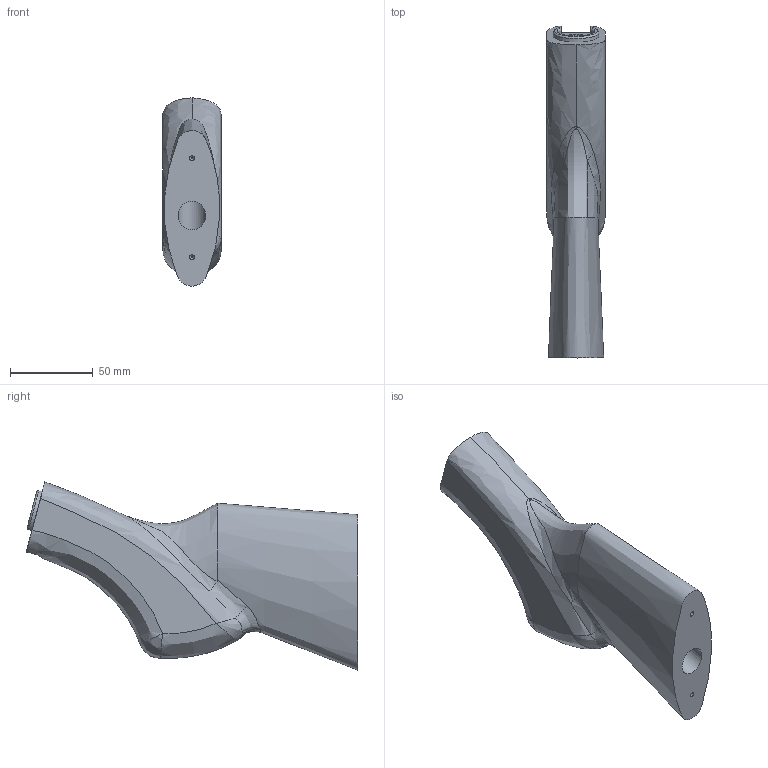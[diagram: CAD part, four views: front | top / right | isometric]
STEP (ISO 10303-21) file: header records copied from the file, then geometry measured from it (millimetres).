
FILE_DESCRIPTION(/* description */ (''),/* implementation_level */ '2;1');
FILE_NAME(/* name */ 'Mare''s Leg Imposter.step',/* time_stamp */ '2022-04-14T02:31:27-04:00',/* author */ (''),/* organization */ (''),/* preprocessor_version */ 'ST-DEVELOPER v18.1',/* originating_system */ 'Autodesk Translation Framework v10.14.0.1471',/* authorisation */ '');
FILE_SCHEMA (('AUTOMOTIVE_DESIGN { 1 0 10303 214 3 1 1 }'));
Length unit declared in the file: millimetre
Products named in the file (1): Mare's Leg Imposter
Bounding box: 35.27 x 201.02 x 113.99 mm (x, y, z)
Volume: 345029 mm3; surface area: 50005.9 mm2
Topology: 1 solids, 1 shells, 59 faces, 152 edges, 94 vertices
Faces by surface type: bspline 31, plane 16, cylinder 8, cone 2, torus 2
Full cylindrical faces by diameter (mm): 2.8 x2, 10 x1, 16.72 x1
Entity records: 5549 total; most frequent: CARTESIAN_POINT 4334, ORIENTED_EDGE 296, DIRECTION 164, EDGE_CURVE 148, VERTEX_POINT 94, B_SPLINE_CURVE_WITH_KNOTS 67, EDGE_LOOP 64, AXIS2_PLACEMENT_3D 63
